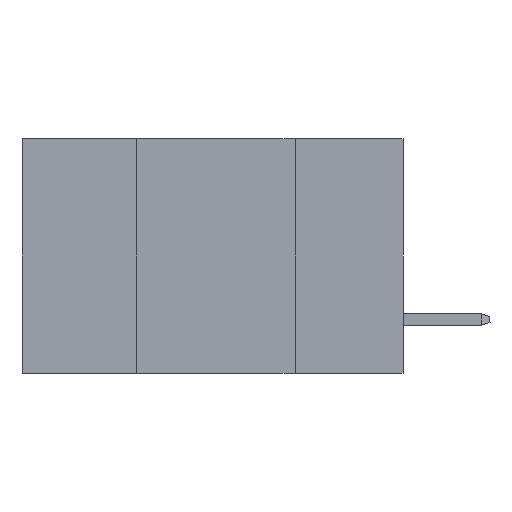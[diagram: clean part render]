
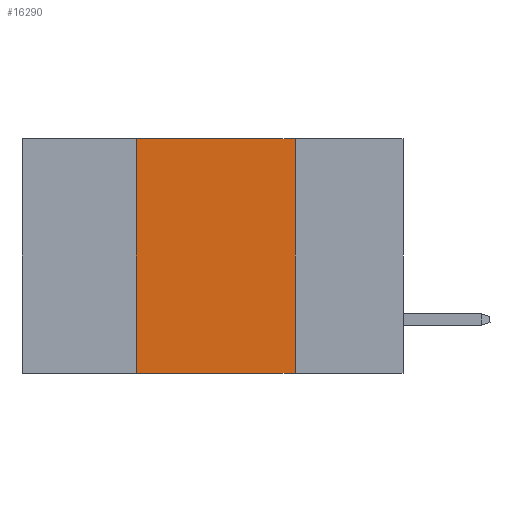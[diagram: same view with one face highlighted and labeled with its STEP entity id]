
A CAD part, left-side view. The second image highlights one B-rep face of the part: STEP entity #16290.
In plain terms, the highlighted planar face has unit normal (-1, 0, 0).
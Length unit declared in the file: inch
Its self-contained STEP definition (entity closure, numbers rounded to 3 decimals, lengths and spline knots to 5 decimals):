
#79 = LINE ( 'NONE', #245, #3963 ) ;
#245 = CARTESIAN_POINT ( 'NONE',  ( 0., 0.42, 0. ) ) ;
#379 = VERTEX_POINT ( 'NONE', #1208 ) ;
#472 = EDGE_CURVE ( 'NONE', #15737, #4485, #79, .T. ) ;
#1030 = VECTOR ( 'NONE', #9391, 39.37008 ) ;
#1114 = FACE_OUTER_BOUND ( 'NONE', #1922, .T. ) ;
#1208 = CARTESIAN_POINT ( 'NONE',  ( 0., 0.17, -0.37 ) ) ;
#1497 = DIRECTION ( 'NONE',  ( 0., 0., 1. ) ) ;
#1922 = EDGE_LOOP ( 'NONE', ( #7468, #2318, #7606, #15542 ) ) ;
#2189 = CARTESIAN_POINT ( 'NONE',  ( 0., 0.17, 0. ) ) ;
#2318 = ORIENTED_EDGE ( 'NONE', *, *, #14600, .F. ) ;
#2867 = LINE ( 'NONE', #8318, #1030 ) ;
#3432 = DIRECTION ( 'NONE',  ( 0., -1., 0. ) ) ;
#3620 = LINE ( 'NONE', #9052, #12751 ) ;
#3963 = VECTOR ( 'NONE', #1497, 39.37008 ) ;
#4485 = VERTEX_POINT ( 'NONE', #13244 ) ;
#4554 = VECTOR ( 'NONE', #13408, 39.37008 ) ;
#5041 = PLANE ( 'NONE',  #14519 ) ;
#6558 = CARTESIAN_POINT ( 'NONE',  ( 0., 0.6, 0. ) ) ;
#6739 = DIRECTION ( 'NONE',  ( 1., 0., 0. ) ) ;
#6933 = CARTESIAN_POINT ( 'NONE',  ( 0., 0.6, -0.37 ) ) ;
#7468 = ORIENTED_EDGE ( 'NONE', *, *, #8725, .F. ) ;
#7606 = ORIENTED_EDGE ( 'NONE', *, *, #472, .F. ) ;
#8099 = VERTEX_POINT ( 'NONE', #2189 ) ;
#8318 = CARTESIAN_POINT ( 'NONE',  ( 0., 0.17, 0. ) ) ;
#8725 = EDGE_CURVE ( 'NONE', #8099, #379, #2867, .T. ) ;
#9052 = CARTESIAN_POINT ( 'NONE',  ( 0., 0.6, 0. ) ) ;
#9391 = DIRECTION ( 'NONE',  ( 0., 0., -1. ) ) ;
#12751 = VECTOR ( 'NONE', #3432, 39.37008 ) ;
#13244 = CARTESIAN_POINT ( 'NONE',  ( 0., 0.42, 0. ) ) ;
#13408 = DIRECTION ( 'NONE',  ( 0., -1., 0. ) ) ;
#13666 = LINE ( 'NONE', #6933, #4554 ) ;
#14519 = AXIS2_PLACEMENT_3D ( 'NONE', #6558, #6739, #16129 ) ;
#14600 = EDGE_CURVE ( 'NONE', #4485, #8099, #3620, .T. ) ;
#15274 = CARTESIAN_POINT ( 'NONE',  ( 0., 0.42, -0.37 ) ) ;
#15542 = ORIENTED_EDGE ( 'NONE', *, *, #15944, .T. ) ;
#15737 = VERTEX_POINT ( 'NONE', #15274 ) ;
#15944 = EDGE_CURVE ( 'NONE', #15737, #379, #13666, .T. ) ;
#16129 = DIRECTION ( 'NONE',  ( 0., 0., -1. ) ) ;
#16290 = ADVANCED_FACE ( 'NONE', ( #1114 ), #5041, .F. ) ;
